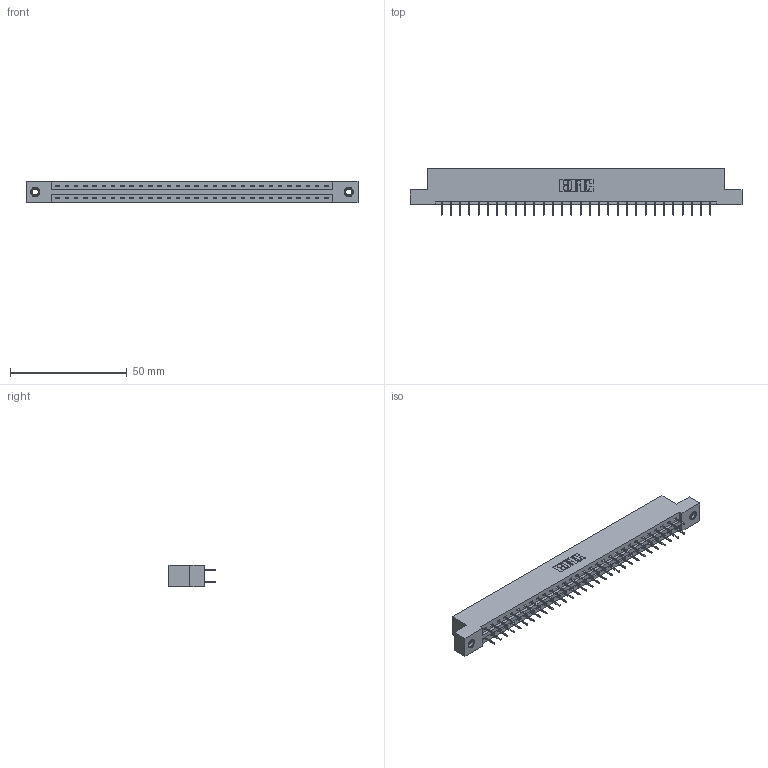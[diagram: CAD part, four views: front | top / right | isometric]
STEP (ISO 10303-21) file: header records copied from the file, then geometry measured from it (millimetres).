
FILE_DESCRIPTION (( 'STEP AP203' ), '1' );
FILE_NAME ('337-060-524-207.STEP', '2018-08-10T07:34:43', ( '' ), ( '' ), 'SwSTEP 2.0', 'SolidWorks 2016', '' );
FILE_SCHEMA (( 'CONFIG_CONTROL_DESIGN' ));
Length unit declared in the file: inch
Products named in the file (4): 337 Part_Flush Mounting Lugs - 0.156 Dia-TI; 345-292-001_345-293-124; 345-250-001_345-250-005-103; 337-060-524-207
Assembly tree (63 placements, depth 2):
  337-060-524-207
    337 Part_Flush Mounting Lugs - 0.156 Dia-TI
    345-292-001_345-293-124  x60
    345-250-001_345-250-005-103  x2
Bounding box: 141.88 x 19.69 x 9.4 mm (x, y, z)
Volume: 14688.9 mm3; surface area: 16243.9 mm2
Topology: 63 solids, 63 shells, 3654 faces, 10347 edges, 6650 vertices
Faces by surface type: plane 2742, cylinder 896, cone 12, torus 4
Entity records: 26072 total; most frequent: CARTESIAN_POINT 4381, ORIENTED_EDGE 4310, DIRECTION 3781, EDGE_CURVE 2155, VECTOR 2011, LINE 2011, VERTEX_POINT 1428, AXIS2_PLACEMENT_3D 885
